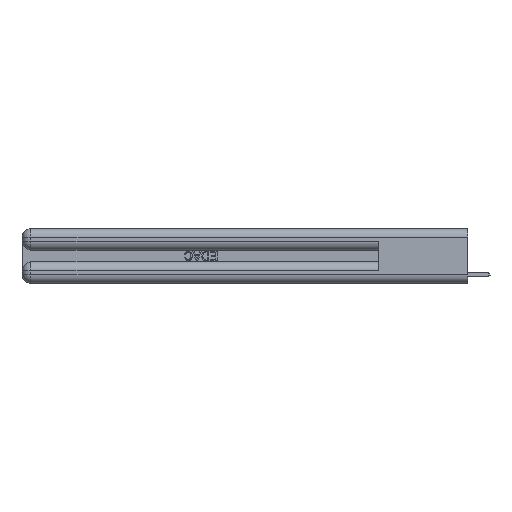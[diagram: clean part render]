
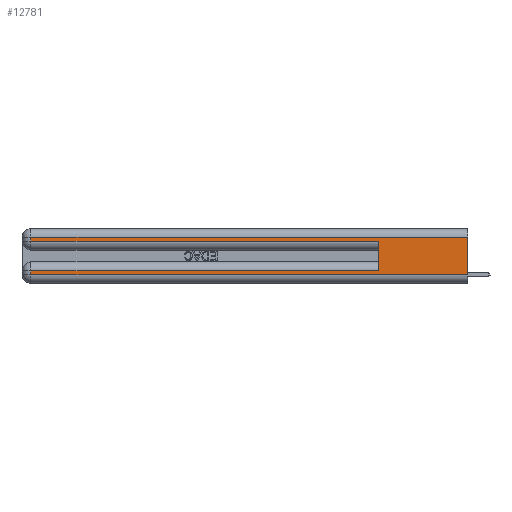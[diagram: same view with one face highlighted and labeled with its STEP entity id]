
A CAD part, left-side view. The second image highlights one B-rep face of the part: STEP entity #12781.
In plain terms, the highlighted planar face has unit normal (-1, 0, 0).
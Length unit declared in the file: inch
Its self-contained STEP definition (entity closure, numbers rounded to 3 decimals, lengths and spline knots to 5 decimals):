
#181 = VERTEX_POINT ( 'NONE', #18933 ) ;
#624 = DIRECTION ( 'NONE',  ( 0., 1., 0. ) ) ;
#861 = DIRECTION ( 'NONE',  ( 0., -1., 0. ) ) ;
#944 = CARTESIAN_POINT ( 'NONE',  ( 0., 0., 0.06 ) ) ;
#1281 = CARTESIAN_POINT ( 'NONE',  ( 0., 0.6, 0.285 ) ) ;
#1340 = PLANE ( 'NONE',  #3369 ) ;
#1372 = CARTESIAN_POINT ( 'NONE',  ( 0., 2.94, 0.31 ) ) ;
#1456 = LINE ( 'NONE', #944, #18853 ) ;
#1633 = VECTOR ( 'NONE', #26701, 39.37008 ) ;
#3324 = ORIENTED_EDGE ( 'NONE', *, *, #15534, .F. ) ;
#3357 = CARTESIAN_POINT ( 'NONE',  ( 0., 0., 0.37 ) ) ;
#3369 = AXIS2_PLACEMENT_3D ( 'NONE', #3357, #18797, #23819 ) ;
#3477 = CARTESIAN_POINT ( 'NONE',  ( 0., 2.94, 0.37 ) ) ;
#3504 = CARTESIAN_POINT ( 'NONE',  ( 0., 2.94, 0.285 ) ) ;
#3961 = VERTEX_POINT ( 'NONE', #32061 ) ;
#4284 = VECTOR ( 'NONE', #25426, 39.37008 ) ;
#4331 = VERTEX_POINT ( 'NONE', #3504 ) ;
#4983 = VECTOR ( 'NONE', #624, 39.37008 ) ;
#5845 = CARTESIAN_POINT ( 'NONE',  ( 0., 0., 0.37 ) ) ;
#6107 = CARTESIAN_POINT ( 'NONE',  ( 0., 2.94, 0.37 ) ) ;
#6322 = LINE ( 'NONE', #18755, #4983 ) ;
#6412 = EDGE_CURVE ( 'NONE', #8337, #4331, #26465, .T. ) ;
#6937 = ORIENTED_EDGE ( 'NONE', *, *, #28347, .T. ) ;
#7467 = LINE ( 'NONE', #18054, #4284 ) ;
#8337 = VERTEX_POINT ( 'NONE', #1372 ) ;
#9689 = EDGE_CURVE ( 'NONE', #3961, #181, #1456, .T. ) ;
#9932 = ORIENTED_EDGE ( 'NONE', *, *, #6412, .T. ) ;
#10130 = EDGE_CURVE ( 'NONE', #10798, #3961, #29101, .T. ) ;
#10798 = VERTEX_POINT ( 'NONE', #22984 ) ;
#11110 = LINE ( 'NONE', #13306, #1633 ) ;
#11361 = DIRECTION ( 'NONE',  ( 0., -1., 0. ) ) ;
#11571 = ORIENTED_EDGE ( 'NONE', *, *, #9689, .T. ) ;
#12781 = ADVANCED_FACE ( 'NONE', ( #14264 ), #1340, .F. ) ;
#12871 = VECTOR ( 'NONE', #861, 39.37008 ) ;
#13080 = DIRECTION ( 'NONE',  ( 0., 0., -1. ) ) ;
#13306 = CARTESIAN_POINT ( 'NONE',  ( 0., 0., 0.085 ) ) ;
#13319 = EDGE_CURVE ( 'NONE', #24618, #8337, #6322, .T. ) ;
#13713 = VECTOR ( 'NONE', #13080, 39.37008 ) ;
#13728 = DIRECTION ( 'NONE',  ( 0., 0., -1. ) ) ;
#14264 = FACE_OUTER_BOUND ( 'NONE', #22925, .T. ) ;
#15534 = EDGE_CURVE ( 'NONE', #24618, #181, #25194, .T. ) ;
#18054 = CARTESIAN_POINT ( 'NONE',  ( 0., 0.6, 0.145 ) ) ;
#18677 = VERTEX_POINT ( 'NONE', #23669 ) ;
#18755 = CARTESIAN_POINT ( 'NONE',  ( 0., 0., 0.31 ) ) ;
#18797 = DIRECTION ( 'NONE',  ( 1., 0., 0. ) ) ;
#18853 = VECTOR ( 'NONE', #11361, 39.37008 ) ;
#18933 = CARTESIAN_POINT ( 'NONE',  ( 0., 0., 0.06 ) ) ;
#19439 = VERTEX_POINT ( 'NONE', #1281 ) ;
#20451 = VECTOR ( 'NONE', #13728, 39.37008 ) ;
#21924 = ORIENTED_EDGE ( 'NONE', *, *, #13319, .T. ) ;
#22925 = EDGE_LOOP ( 'NONE', ( #3324, #21924, #9932, #6937, #26824, #24327, #30025, #11571 ) ) ;
#22984 = CARTESIAN_POINT ( 'NONE',  ( 0., 2.94, 0.085 ) ) ;
#23669 = CARTESIAN_POINT ( 'NONE',  ( 0., 0.6, 0.085 ) ) ;
#23819 = DIRECTION ( 'NONE',  ( 0., 0., -1. ) ) ;
#24327 = ORIENTED_EDGE ( 'NONE', *, *, #28444, .T. ) ;
#24618 = VERTEX_POINT ( 'NONE', #27694 ) ;
#25194 = LINE ( 'NONE', #5845, #13713 ) ;
#25426 = DIRECTION ( 'NONE',  ( 0., 0., 1. ) ) ;
#26465 = LINE ( 'NONE', #3477, #20451 ) ;
#26580 = DIRECTION ( 'NONE',  ( 0., 0., -1. ) ) ;
#26701 = DIRECTION ( 'NONE',  ( 0., 1., 0. ) ) ;
#26824 = ORIENTED_EDGE ( 'NONE', *, *, #27968, .F. ) ;
#27694 = CARTESIAN_POINT ( 'NONE',  ( 0., 0., 0.31 ) ) ;
#27968 = EDGE_CURVE ( 'NONE', #18677, #19439, #7467, .T. ) ;
#28347 = EDGE_CURVE ( 'NONE', #4331, #19439, #28899, .T. ) ;
#28444 = EDGE_CURVE ( 'NONE', #18677, #10798, #11110, .T. ) ;
#28507 = VECTOR ( 'NONE', #26580, 39.37008 ) ;
#28899 = LINE ( 'NONE', #31742, #12871 ) ;
#29101 = LINE ( 'NONE', #6107, #28507 ) ;
#30025 = ORIENTED_EDGE ( 'NONE', *, *, #10130, .T. ) ;
#31742 = CARTESIAN_POINT ( 'NONE',  ( 0., 0., 0.285 ) ) ;
#32061 = CARTESIAN_POINT ( 'NONE',  ( 0., 2.94, 0.06 ) ) ;
